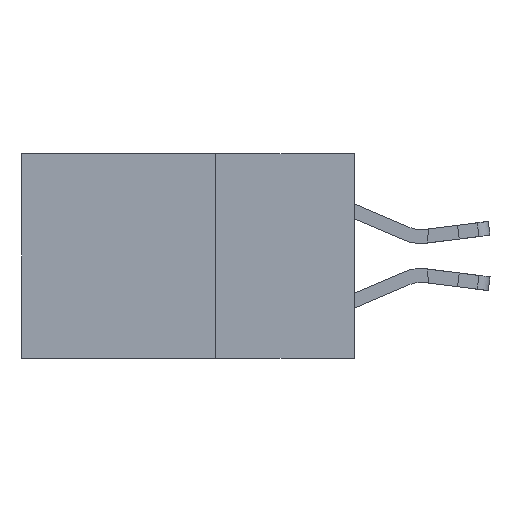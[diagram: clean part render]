
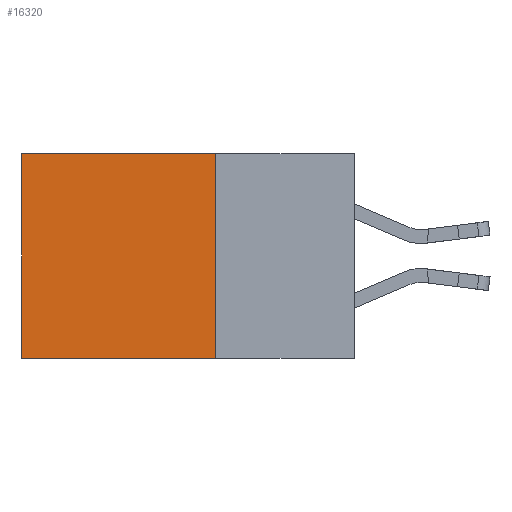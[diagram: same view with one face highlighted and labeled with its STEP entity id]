
A CAD part, left-side view. The second image highlights one B-rep face of the part: STEP entity #16320.
In plain terms, the highlighted planar face has unit normal (-1, 0, 0).
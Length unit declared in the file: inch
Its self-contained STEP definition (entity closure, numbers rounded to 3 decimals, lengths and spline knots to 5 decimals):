
#1224 = CARTESIAN_POINT ( 'NONE',  ( 0.298, 0.25, 0. ) ) ;
#1293 = DIRECTION ( 'NONE',  ( 0., 0., -1. ) ) ;
#3245 = DIRECTION ( 'NONE',  ( 0., 1., 0. ) ) ;
#3541 = ORIENTED_EDGE ( 'NONE', *, *, #4463, .T. ) ;
#4262 = VECTOR ( 'NONE', #5552, 39.37008 ) ;
#4463 = EDGE_CURVE ( 'NONE', #15918, #8667, #14783, .T. ) ;
#4593 = DIRECTION ( 'NONE',  ( 1., 0., 0. ) ) ;
#4642 = LINE ( 'NONE', #1224, #10784 ) ;
#4868 = CARTESIAN_POINT ( 'NONE',  ( 0.298, 0.25, 0. ) ) ;
#5079 = FACE_OUTER_BOUND ( 'NONE', #13233, .T. ) ;
#5100 = CARTESIAN_POINT ( 'NONE',  ( 0.298, 0.6, 0. ) ) ;
#5552 = DIRECTION ( 'NONE',  ( 0., 1., 0. ) ) ;
#6088 = DIRECTION ( 'NONE',  ( 0., 0., -1. ) ) ;
#8667 = VERTEX_POINT ( 'NONE', #5100 ) ;
#8693 = ORIENTED_EDGE ( 'NONE', *, *, #18797, .T. ) ;
#9322 = ORIENTED_EDGE ( 'NONE', *, *, #19951, .F. ) ;
#9805 = CARTESIAN_POINT ( 'NONE',  ( 0.298, 0.25, -0.37 ) ) ;
#10694 = EDGE_CURVE ( 'NONE', #14396, #19291, #19332, .T. ) ;
#10784 = VECTOR ( 'NONE', #1293, 39.37008 ) ;
#12771 = CARTESIAN_POINT ( 'NONE',  ( 0.298, 0.6, 0. ) ) ;
#13022 = CARTESIAN_POINT ( 'NONE',  ( 0.298, 0.25, -0.37 ) ) ;
#13233 = EDGE_LOOP ( 'NONE', ( #8693, #14144, #9322, #3541 ) ) ;
#14144 = ORIENTED_EDGE ( 'NONE', *, *, #10694, .F. ) ;
#14336 = PLANE ( 'NONE',  #14713 ) ;
#14396 = VERTEX_POINT ( 'NONE', #9805 ) ;
#14644 = CARTESIAN_POINT ( 'NONE',  ( 0.298, 0.6, -0.37 ) ) ;
#14713 = AXIS2_PLACEMENT_3D ( 'NONE', #15826, #4593, #6088 ) ;
#14783 = LINE ( 'NONE', #16983, #4262 ) ;
#15826 = CARTESIAN_POINT ( 'NONE',  ( 0.298, 0.25, 0. ) ) ;
#15918 = VERTEX_POINT ( 'NONE', #4868 ) ;
#16320 = ADVANCED_FACE ( 'NONE', ( #5079 ), #14336, .F. ) ;
#16983 = CARTESIAN_POINT ( 'NONE',  ( 0.298, 0.25, 0. ) ) ;
#17545 = DIRECTION ( 'NONE',  ( 0., 0., -1. ) ) ;
#18797 = EDGE_CURVE ( 'NONE', #8667, #19291, #20859, .T. ) ;
#19291 = VERTEX_POINT ( 'NONE', #14644 ) ;
#19332 = LINE ( 'NONE', #13022, #20625 ) ;
#19951 = EDGE_CURVE ( 'NONE', #15918, #14396, #4642, .T. ) ;
#20097 = VECTOR ( 'NONE', #17545, 39.37008 ) ;
#20625 = VECTOR ( 'NONE', #3245, 39.37008 ) ;
#20859 = LINE ( 'NONE', #12771, #20097 ) ;
